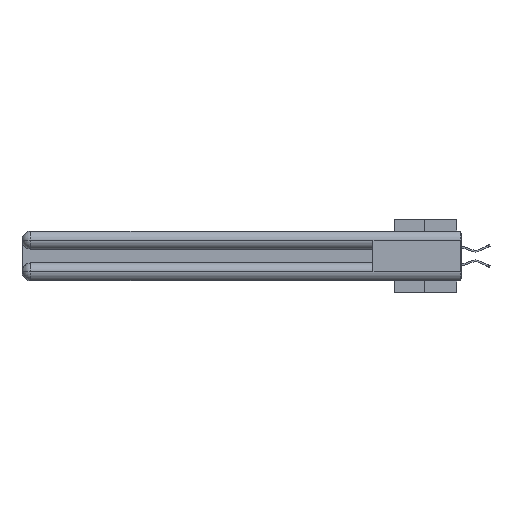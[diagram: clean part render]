
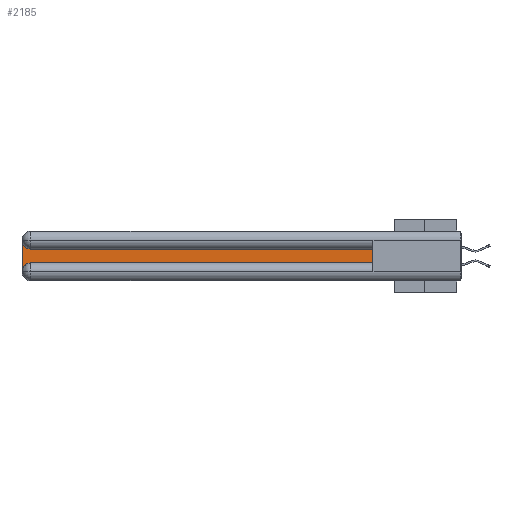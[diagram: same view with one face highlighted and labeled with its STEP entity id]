
A CAD part, left-side view. The second image highlights one B-rep face of the part: STEP entity #2185.
In plain terms, the highlighted planar face has unit normal (-1, 0, 0).
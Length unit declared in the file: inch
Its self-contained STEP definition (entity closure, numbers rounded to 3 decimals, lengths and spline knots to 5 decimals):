
#122 = CARTESIAN_POINT ( 'NONE',  ( 0.075, 3., -0.0625 ) ) ;
#542 = LINE ( 'NONE', #8304, #7924 ) ;
#1847 = VECTOR ( 'NONE', #10096, 39.37008 ) ;
#2185 = ADVANCED_FACE ( 'NONE', ( #32983 ), #18263, .F. ) ;
#2312 = DIRECTION ( 'NONE',  ( 1., 0., 0. ) ) ;
#2408 = CARTESIAN_POINT ( 'NONE',  ( 0.075, 3., -0.2775 ) ) ;
#3340 = CARTESIAN_POINT ( 'NONE',  ( 0.075, 3., -0.1225 ) ) ;
#3799 = LINE ( 'NONE', #6146, #13162 ) ;
#4376 = CIRCLE ( 'NONE', #20251, 0.06 ) ;
#5386 = EDGE_CURVE ( 'NONE', #34454, #36848, #27783, .T. ) ;
#6146 = CARTESIAN_POINT ( 'NONE',  ( 0.075, 0.6, -0.2175 ) ) ;
#7199 = EDGE_CURVE ( 'NONE', #32350, #34454, #32974, .T. ) ;
#7458 = AXIS2_PLACEMENT_3D ( 'NONE', #21131, #18101, #21261 ) ;
#7471 = VERTEX_POINT ( 'NONE', #22582 ) ;
#7654 = EDGE_CURVE ( 'NONE', #36848, #8696, #542, .T. ) ;
#7702 = ORIENTED_EDGE ( 'NONE', *, *, #32675, .T. ) ;
#7924 = VECTOR ( 'NONE', #11678, 39.37008 ) ;
#8260 = DIRECTION ( 'NONE',  ( 0., 0., -1. ) ) ;
#8304 = CARTESIAN_POINT ( 'NONE',  ( 0.075, 0.6, -0.2175 ) ) ;
#8696 = VERTEX_POINT ( 'NONE', #33025 ) ;
#9142 = DIRECTION ( 'NONE',  ( 0., 0., 1. ) ) ;
#10013 = EDGE_CURVE ( 'NONE', #32621, #7471, #39172, .T. ) ;
#10096 = DIRECTION ( 'NONE',  ( 0., 1., 0. ) ) ;
#10295 = DIRECTION ( 'NONE',  ( 0., 0., -1. ) ) ;
#11678 = DIRECTION ( 'NONE',  ( 0., -1., 0. ) ) ;
#12069 = ORIENTED_EDGE ( 'NONE', *, *, #10013, .T. ) ;
#12090 = ORIENTED_EDGE ( 'NONE', *, *, #29600, .T. ) ;
#13128 = CARTESIAN_POINT ( 'NONE',  ( 0.075, 0.6, -0.1225 ) ) ;
#13162 = VECTOR ( 'NONE', #9142, 39.37008 ) ;
#14301 = ORIENTED_EDGE ( 'NONE', *, *, #5386, .T. ) ;
#15794 = CARTESIAN_POINT ( 'NONE',  ( 0.075, 2.94, -0.2175 ) ) ;
#16955 = EDGE_LOOP ( 'NONE', ( #12069, #12090, #38524, #14301, #20423, #7702 ) ) ;
#18101 = DIRECTION ( 'NONE',  ( 1., 0., 0. ) ) ;
#18263 = PLANE ( 'NONE',  #28637 ) ;
#20251 = AXIS2_PLACEMENT_3D ( 'NONE', #33868, #2312, #8260 ) ;
#20423 = ORIENTED_EDGE ( 'NONE', *, *, #7654, .T. ) ;
#21131 = CARTESIAN_POINT ( 'NONE',  ( 0.075, 2.94, -0.2775 ) ) ;
#21261 = DIRECTION ( 'NONE',  ( 0., 0., -1. ) ) ;
#21980 = DIRECTION ( 'NONE',  ( 0., 0., -1. ) ) ;
#22582 = CARTESIAN_POINT ( 'NONE',  ( 0.075, 2.94, -0.1225 ) ) ;
#24475 = CARTESIAN_POINT ( 'NONE',  ( 0.075, 0.6, -0.1225 ) ) ;
#25390 = DIRECTION ( 'NONE',  ( 1., 0., 0. ) ) ;
#26589 = VECTOR ( 'NONE', #10295, 39.37008 ) ;
#27783 = CIRCLE ( 'NONE', #7458, 0.06 ) ;
#28637 = AXIS2_PLACEMENT_3D ( 'NONE', #3340, #25390, #21980 ) ;
#29600 = EDGE_CURVE ( 'NONE', #7471, #32350, #4376, .T. ) ;
#32350 = VERTEX_POINT ( 'NONE', #122 ) ;
#32359 = CARTESIAN_POINT ( 'NONE',  ( 0.075, 3., -0.2175 ) ) ;
#32621 = VERTEX_POINT ( 'NONE', #24475 ) ;
#32675 = EDGE_CURVE ( 'NONE', #8696, #32621, #3799, .T. ) ;
#32974 = LINE ( 'NONE', #32359, #26589 ) ;
#32983 = FACE_OUTER_BOUND ( 'NONE', #16955, .T. ) ;
#33025 = CARTESIAN_POINT ( 'NONE',  ( 0.075, 0.6, -0.2175 ) ) ;
#33868 = CARTESIAN_POINT ( 'NONE',  ( 0.075, 2.94, -0.0625 ) ) ;
#34454 = VERTEX_POINT ( 'NONE', #2408 ) ;
#36848 = VERTEX_POINT ( 'NONE', #15794 ) ;
#38524 = ORIENTED_EDGE ( 'NONE', *, *, #7199, .T. ) ;
#39172 = LINE ( 'NONE', #13128, #1847 ) ;
